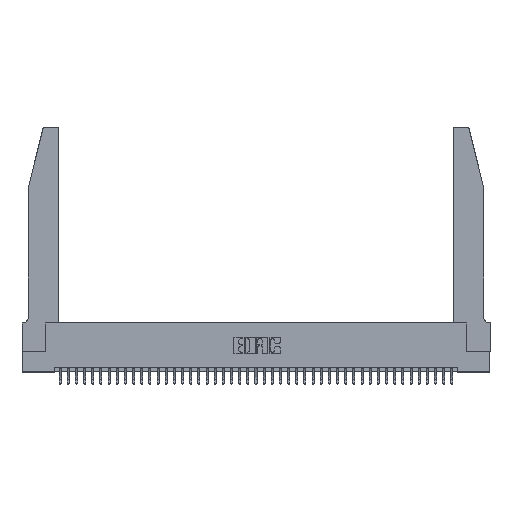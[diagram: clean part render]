
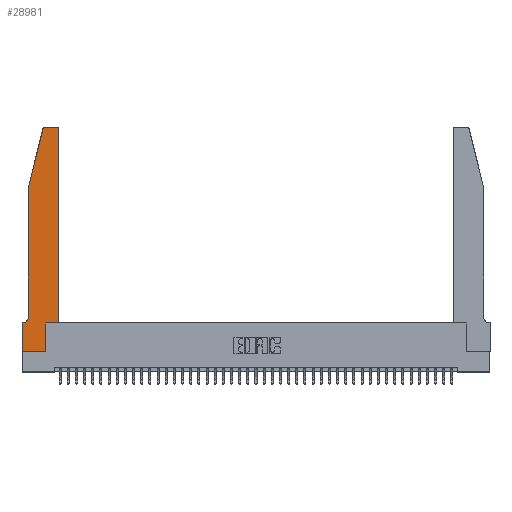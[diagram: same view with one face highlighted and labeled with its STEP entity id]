
A CAD part, top view. The second image highlights one B-rep face of the part: STEP entity #28981.
In plain terms, the highlighted planar face has unit normal (0, 0, 1).
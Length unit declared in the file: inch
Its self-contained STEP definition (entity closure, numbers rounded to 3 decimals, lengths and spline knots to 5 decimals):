
#50 = LINE ( 'NONE', #19211, #25364 ) ;
#260 = CARTESIAN_POINT ( 'NONE',  ( 0.4505, 0.35, 0.37 ) ) ;
#626 = DIRECTION ( 'NONE',  ( 1., 0., 0. ) ) ;
#854 = EDGE_CURVE ( 'NONE', #32585, #26520, #15168, .T. ) ;
#925 = ORIENTED_EDGE ( 'NONE', *, *, #3714, .T. ) ;
#1317 = DIRECTION ( 'NONE',  ( -1., 0., 0. ) ) ;
#1411 = DIRECTION ( 'NONE',  ( 1., 0., 0. ) ) ;
#1506 = VECTOR ( 'NONE', #17274, 39.37008 ) ;
#1949 = CARTESIAN_POINT ( 'NONE',  ( 0.4505, 0.35, 0.37 ) ) ;
#3288 = ORIENTED_EDGE ( 'NONE', *, *, #17987, .T. ) ;
#3352 = ORIENTED_EDGE ( 'NONE', *, *, #9688, .T. ) ;
#3714 = EDGE_CURVE ( 'NONE', #10021, #4970, #23468, .T. ) ;
#3873 = ORIENTED_EDGE ( 'NONE', *, *, #40203, .T. ) ;
#3953 = CARTESIAN_POINT ( 'NONE',  ( 0.2865, 0.35, 0.37 ) ) ;
#4693 = ORIENTED_EDGE ( 'NONE', *, *, #32491, .T. ) ;
#4970 = VERTEX_POINT ( 'NONE', #41932 ) ;
#5404 = LINE ( 'NONE', #260, #13163 ) ;
#5868 = VECTOR ( 'NONE', #25047, 39.37008 ) ;
#6064 = ORIENTED_EDGE ( 'NONE', *, *, #32807, .T. ) ;
#6602 = EDGE_CURVE ( 'NONE', #26520, #10066, #10293, .T. ) ;
#7146 = DIRECTION ( 'NONE',  ( 0., -1., 0. ) ) ;
#7505 = CARTESIAN_POINT ( 'NONE',  ( 0.4505, 2.72, 0.37 ) ) ;
#7576 = LINE ( 'NONE', #26891, #24109 ) ;
#8187 = FACE_OUTER_BOUND ( 'NONE', #36011, .T. ) ;
#8218 = CARTESIAN_POINT ( 'NONE',  ( 0.0755, 0.35, 0.37 ) ) ;
#8550 = VERTEX_POINT ( 'NONE', #19152 ) ;
#9127 = ORIENTED_EDGE ( 'NONE', *, *, #854, .T. ) ;
#9194 = ORIENTED_EDGE ( 'NONE', *, *, #28726, .T. ) ;
#9688 = EDGE_CURVE ( 'NONE', #16434, #28799, #12152, .T. ) ;
#10021 = VERTEX_POINT ( 'NONE', #39771 ) ;
#10066 = VERTEX_POINT ( 'NONE', #36662 ) ;
#10227 = ORIENTED_EDGE ( 'NONE', *, *, #23671, .T. ) ;
#10293 = LINE ( 'NONE', #3953, #1506 ) ;
#11171 = CARTESIAN_POINT ( 'NONE',  ( 0.4505, 0.35, 0.37 ) ) ;
#11530 = DIRECTION ( 'NONE',  ( -1., 0., 0. ) ) ;
#12152 = CIRCLE ( 'NONE', #22472, 0.03 ) ;
#12720 = EDGE_CURVE ( 'NONE', #10066, #42017, #14673, .T. ) ;
#12859 = DIRECTION ( 'NONE',  ( 0., -1., 0. ) ) ;
#13040 = CIRCLE ( 'NONE', #33537, 0.07 ) ;
#13163 = VECTOR ( 'NONE', #39606, 39.37008 ) ;
#13676 = CARTESIAN_POINT ( 'NONE',  ( 0.4205, 2.75, 0.37 ) ) ;
#14415 = PLANE ( 'NONE',  #39462 ) ;
#14673 = LINE ( 'NONE', #1949, #5868 ) ;
#15168 = LINE ( 'NONE', #29257, #25414 ) ;
#15209 = CARTESIAN_POINT ( 'NONE',  ( 0.2865, 0., 0.37 ) ) ;
#16016 = ORIENTED_EDGE ( 'NONE', *, *, #21583, .T. ) ;
#16088 = VERTEX_POINT ( 'NONE', #35395 ) ;
#16434 = VERTEX_POINT ( 'NONE', #7505 ) ;
#17150 = VECTOR ( 'NONE', #32518, 39.37008 ) ;
#17274 = DIRECTION ( 'NONE',  ( 0., 1., 0. ) ) ;
#17987 = EDGE_CURVE ( 'NONE', #28799, #10021, #40987, .T. ) ;
#18507 = CARTESIAN_POINT ( 'NONE',  ( 0.4205, 2.72, 0.37 ) ) ;
#19152 = CARTESIAN_POINT ( 'NONE',  ( 0., 0.35, 0.37 ) ) ;
#19211 = CARTESIAN_POINT ( 'NONE',  ( 0.0755, 2., 0.37 ) ) ;
#19854 = CARTESIAN_POINT ( 'NONE',  ( 0.0755, 0.42, 0.37 ) ) ;
#20418 = DIRECTION ( 'NONE',  ( 0., 0., 1. ) ) ;
#21116 = DIRECTION ( 'NONE',  ( 0., 0., -1. ) ) ;
#21199 = DIRECTION ( 'NONE',  ( 0., 0., 1. ) ) ;
#21583 = EDGE_CURVE ( 'NONE', #26624, #26105, #50, .T. ) ;
#21849 = DIRECTION ( 'NONE',  ( 1., 0., 0. ) ) ;
#22472 = AXIS2_PLACEMENT_3D ( 'NONE', #18507, #41365, #21849 ) ;
#22625 = VECTOR ( 'NONE', #25513, 39.37008 ) ;
#23468 = CIRCLE ( 'NONE', #37535, 0.03 ) ;
#23671 = EDGE_CURVE ( 'NONE', #16088, #8550, #32574, .T. ) ;
#24109 = VECTOR ( 'NONE', #7146, 39.37008 ) ;
#25047 = DIRECTION ( 'NONE',  ( 1., 0., 0. ) ) ;
#25364 = VECTOR ( 'NONE', #12859, 39.37008 ) ;
#25414 = VECTOR ( 'NONE', #32522, 39.37008 ) ;
#25513 = DIRECTION ( 'NONE',  ( -1., 0., 0. ) ) ;
#25574 = CARTESIAN_POINT ( 'NONE',  ( 0.0755, 2., 0.37 ) ) ;
#26105 = VERTEX_POINT ( 'NONE', #19854 ) ;
#26520 = VERTEX_POINT ( 'NONE', #15209 ) ;
#26624 = VERTEX_POINT ( 'NONE', #25574 ) ;
#26891 = CARTESIAN_POINT ( 'NONE',  ( 0., 0., 0.37 ) ) ;
#28726 = EDGE_CURVE ( 'NONE', #42017, #16434, #5404, .T. ) ;
#28799 = VERTEX_POINT ( 'NONE', #13676 ) ;
#28981 = ADVANCED_FACE ( 'NONE', ( #8187 ), #14415, .T. ) ;
#29251 = CARTESIAN_POINT ( 'NONE',  ( 0.0755, 2., 0.37 ) ) ;
#29257 = CARTESIAN_POINT ( 'NONE',  ( 0., 0., 0.37 ) ) ;
#31253 = CARTESIAN_POINT ( 'NONE',  ( 0., 0., 0.37 ) ) ;
#32491 = EDGE_CURVE ( 'NONE', #26105, #16088, #13040, .T. ) ;
#32518 = DIRECTION ( 'NONE',  ( -0.239, -0.971, 0. ) ) ;
#32522 = DIRECTION ( 'NONE',  ( 1., 0., 0. ) ) ;
#32574 = LINE ( 'NONE', #8218, #41221 ) ;
#32585 = VERTEX_POINT ( 'NONE', #31253 ) ;
#32807 = EDGE_CURVE ( 'NONE', #4970, #26624, #34561, .T. ) ;
#33537 = AXIS2_PLACEMENT_3D ( 'NONE', #40648, #21116, #1317 ) ;
#34561 = LINE ( 'NONE', #29251, #17150 ) ;
#35395 = CARTESIAN_POINT ( 'NONE',  ( 0.0055, 0.35, 0.37 ) ) ;
#35938 = ORIENTED_EDGE ( 'NONE', *, *, #12720, .T. ) ;
#36011 = EDGE_LOOP ( 'NONE', ( #3288, #925, #6064, #16016, #4693, #10227, #3873, #9127, #37752, #35938, #9194, #3352 ) ) ;
#36662 = CARTESIAN_POINT ( 'NONE',  ( 0.2865, 0.35, 0.37 ) ) ;
#37465 = CARTESIAN_POINT ( 'NONE',  ( 0., 0.35, 0.37 ) ) ;
#37535 = AXIS2_PLACEMENT_3D ( 'NONE', #39966, #20418, #626 ) ;
#37752 = ORIENTED_EDGE ( 'NONE', *, *, #6602, .T. ) ;
#38616 = CARTESIAN_POINT ( 'NONE',  ( 0.2605, 2.75, 0.37 ) ) ;
#39462 = AXIS2_PLACEMENT_3D ( 'NONE', #37465, #21199, #1411 ) ;
#39606 = DIRECTION ( 'NONE',  ( 0., 1., 0. ) ) ;
#39771 = CARTESIAN_POINT ( 'NONE',  ( 0.284, 2.75, 0.37 ) ) ;
#39966 = CARTESIAN_POINT ( 'NONE',  ( 0.284, 2.72, 0.37 ) ) ;
#40203 = EDGE_CURVE ( 'NONE', #8550, #32585, #7576, .T. ) ;
#40648 = CARTESIAN_POINT ( 'NONE',  ( 0.0055, 0.42, 0.37 ) ) ;
#40987 = LINE ( 'NONE', #38616, #22625 ) ;
#41221 = VECTOR ( 'NONE', #11530, 39.37008 ) ;
#41365 = DIRECTION ( 'NONE',  ( 0., 0., 1. ) ) ;
#41932 = CARTESIAN_POINT ( 'NONE',  ( 0.25487, 2.72718, 0.37 ) ) ;
#42017 = VERTEX_POINT ( 'NONE', #11171 ) ;
